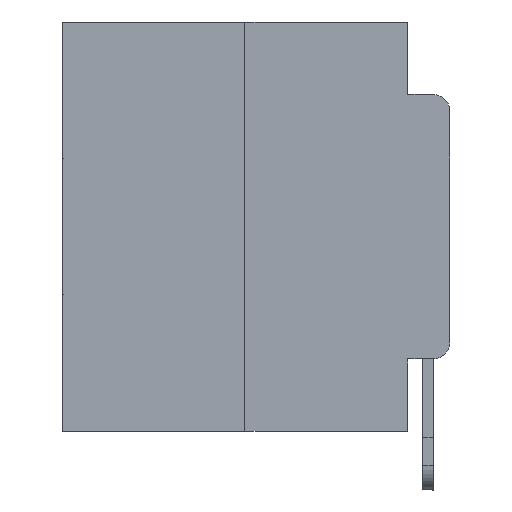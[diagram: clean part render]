
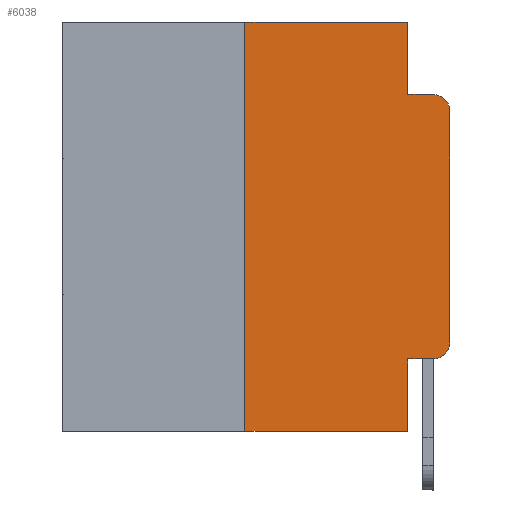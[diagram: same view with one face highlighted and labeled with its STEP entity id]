
A CAD part, left-side view. The second image highlights one B-rep face of the part: STEP entity #6038.
In plain terms, the highlighted planar face has unit normal (-1, 0, 0).
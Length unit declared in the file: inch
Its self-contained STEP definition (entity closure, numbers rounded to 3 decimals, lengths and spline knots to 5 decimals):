
#19 = CARTESIAN_POINT ( 'NONE',  ( 0., 0., -0.3915 ) ) ;
#125 = EDGE_CURVE ( 'NONE', #15231, #26801, #13646, .T. ) ;
#130 = ORIENTED_EDGE ( 'NONE', *, *, #26424, .F. ) ;
#400 = ORIENTED_EDGE ( 'NONE', *, *, #14389, .F. ) ;
#762 = VECTOR ( 'NONE', #23208, 39.37008 ) ;
#791 = EDGE_CURVE ( 'NONE', #6172, #15231, #17228, .T. ) ;
#1252 = AXIS2_PLACEMENT_3D ( 'NONE', #3411, #26337, #20342 ) ;
#2015 = ORIENTED_EDGE ( 'NONE', *, *, #16376, .T. ) ;
#2365 = EDGE_CURVE ( 'NONE', #19138, #3930, #10158, .T. ) ;
#2474 = EDGE_LOOP ( 'NONE', ( #2015, #10933, #130, #400, #17332, #11051, #21957, #4790, #17585, #7197 ) ) ;
#2741 = CARTESIAN_POINT ( 'NONE',  ( 0., 0.051, -0.0885 ) ) ;
#3411 = CARTESIAN_POINT ( 'NONE',  ( 0., 0.02, -0.3915 ) ) ;
#3903 = CARTESIAN_POINT ( 'NONE',  ( 0., 0.25, 0. ) ) ;
#3930 = VERTEX_POINT ( 'NONE', #11293 ) ;
#3975 = DIRECTION ( 'NONE',  ( 0., 0., -1. ) ) ;
#4408 = DIRECTION ( 'NONE',  ( 0., 0., -1. ) ) ;
#4790 = ORIENTED_EDGE ( 'NONE', *, *, #7098, .F. ) ;
#4988 = CARTESIAN_POINT ( 'NONE',  ( 0., 0.051, 0. ) ) ;
#5532 = EDGE_CURVE ( 'NONE', #17738, #21422, #14128, .T. ) ;
#5907 = VERTEX_POINT ( 'NONE', #2741 ) ;
#5915 = VECTOR ( 'NONE', #3975, 39.37008 ) ;
#6038 = ADVANCED_FACE ( 'NONE', ( #24788 ), #26748, .F. ) ;
#6126 = CARTESIAN_POINT ( 'NONE',  ( 0., 0.473, 0. ) ) ;
#6172 = VERTEX_POINT ( 'NONE', #10348 ) ;
#6527 = VECTOR ( 'NONE', #18890, 39.37008 ) ;
#7098 = EDGE_CURVE ( 'NONE', #6172, #21422, #19699, .T. ) ;
#7131 = LINE ( 'NONE', #11570, #13548 ) ;
#7197 = ORIENTED_EDGE ( 'NONE', *, *, #125, .T. ) ;
#7368 = CARTESIAN_POINT ( 'NONE',  ( 0., 0.051, -0.5 ) ) ;
#7539 = DIRECTION ( 'NONE',  ( 0., 0., 1. ) ) ;
#7619 = CARTESIAN_POINT ( 'NONE',  ( 0., 0.473, -0.5 ) ) ;
#7714 = DIRECTION ( 'NONE',  ( 0., 0., -1. ) ) ;
#8199 = AXIS2_PLACEMENT_3D ( 'NONE', #16456, #11747, #7714 ) ;
#10158 = LINE ( 'NONE', #6126, #11543 ) ;
#10304 = EDGE_CURVE ( 'NONE', #17738, #19138, #22917, .T. ) ;
#10348 = CARTESIAN_POINT ( 'NONE',  ( 0., 0.051, -0.4115 ) ) ;
#10824 = DIRECTION ( 'NONE',  ( 0., 0., -1. ) ) ;
#10933 = ORIENTED_EDGE ( 'NONE', *, *, #23420, .T. ) ;
#11051 = ORIENTED_EDGE ( 'NONE', *, *, #10304, .F. ) ;
#11293 = CARTESIAN_POINT ( 'NONE',  ( 0., 0.051, 0. ) ) ;
#11543 = VECTOR ( 'NONE', #14595, 39.37008 ) ;
#11570 = CARTESIAN_POINT ( 'NONE',  ( 0., 0., 0. ) ) ;
#11747 = DIRECTION ( 'NONE',  ( 1., 0., 0. ) ) ;
#12239 = CARTESIAN_POINT ( 'NONE',  ( 0., 0.02, -0.4115 ) ) ;
#12744 = CARTESIAN_POINT ( 'NONE',  ( 0., 0.02, -0.1085 ) ) ;
#13548 = VECTOR ( 'NONE', #7539, 39.37008 ) ;
#13646 = CIRCLE ( 'NONE', #1252, 0.02 ) ;
#14128 = LINE ( 'NONE', #7619, #15225 ) ;
#14201 = VERTEX_POINT ( 'NONE', #22021 ) ;
#14389 = EDGE_CURVE ( 'NONE', #3930, #5907, #25078, .T. ) ;
#14595 = DIRECTION ( 'NONE',  ( 0., -1., 0. ) ) ;
#14788 = CARTESIAN_POINT ( 'NONE',  ( 0., 0.25, -0.5 ) ) ;
#15225 = VECTOR ( 'NONE', #16216, 39.37008 ) ;
#15231 = VERTEX_POINT ( 'NONE', #12239 ) ;
#16216 = DIRECTION ( 'NONE',  ( 0., -1., 0. ) ) ;
#16376 = EDGE_CURVE ( 'NONE', #26801, #14201, #7131, .T. ) ;
#16456 = CARTESIAN_POINT ( 'NONE',  ( 0., 0.473, 0. ) ) ;
#17228 = LINE ( 'NONE', #23340, #20359 ) ;
#17332 = ORIENTED_EDGE ( 'NONE', *, *, #2365, .F. ) ;
#17585 = ORIENTED_EDGE ( 'NONE', *, *, #791, .T. ) ;
#17738 = VERTEX_POINT ( 'NONE', #14788 ) ;
#18627 = LINE ( 'NONE', #27112, #762 ) ;
#18890 = DIRECTION ( 'NONE',  ( 0., 0., 1. ) ) ;
#19138 = VERTEX_POINT ( 'NONE', #23803 ) ;
#19486 = CIRCLE ( 'NONE', #23041, 0.02 ) ;
#19699 = LINE ( 'NONE', #4988, #22970 ) ;
#20307 = CARTESIAN_POINT ( 'NONE',  ( 0., 0.02, -0.0885 ) ) ;
#20342 = DIRECTION ( 'NONE',  ( 0., 0., -1. ) ) ;
#20359 = VECTOR ( 'NONE', #21267, 39.37008 ) ;
#21267 = DIRECTION ( 'NONE',  ( 0., -1., 0. ) ) ;
#21422 = VERTEX_POINT ( 'NONE', #7368 ) ;
#21957 = ORIENTED_EDGE ( 'NONE', *, *, #5532, .T. ) ;
#22021 = CARTESIAN_POINT ( 'NONE',  ( 0., 0., -0.1085 ) ) ;
#22917 = LINE ( 'NONE', #3903, #6527 ) ;
#22970 = VECTOR ( 'NONE', #10824, 39.37008 ) ;
#22989 = CARTESIAN_POINT ( 'NONE',  ( 0., 0.051, 0. ) ) ;
#23041 = AXIS2_PLACEMENT_3D ( 'NONE', #12744, #23685, #4408 ) ;
#23208 = DIRECTION ( 'NONE',  ( 0., -1., 0. ) ) ;
#23340 = CARTESIAN_POINT ( 'NONE',  ( 0., 0.051, -0.4115 ) ) ;
#23420 = EDGE_CURVE ( 'NONE', #14201, #25088, #19486, .T. ) ;
#23685 = DIRECTION ( 'NONE',  ( -1., 0., 0. ) ) ;
#23803 = CARTESIAN_POINT ( 'NONE',  ( 0., 0.25, 0. ) ) ;
#24788 = FACE_OUTER_BOUND ( 'NONE', #2474, .T. ) ;
#25078 = LINE ( 'NONE', #22989, #5915 ) ;
#25088 = VERTEX_POINT ( 'NONE', #20307 ) ;
#26337 = DIRECTION ( 'NONE',  ( -1., 0., 0. ) ) ;
#26424 = EDGE_CURVE ( 'NONE', #5907, #25088, #18627, .T. ) ;
#26748 = PLANE ( 'NONE',  #8199 ) ;
#26801 = VERTEX_POINT ( 'NONE', #19 ) ;
#27112 = CARTESIAN_POINT ( 'NONE',  ( 0., 0.051, -0.0885 ) ) ;
